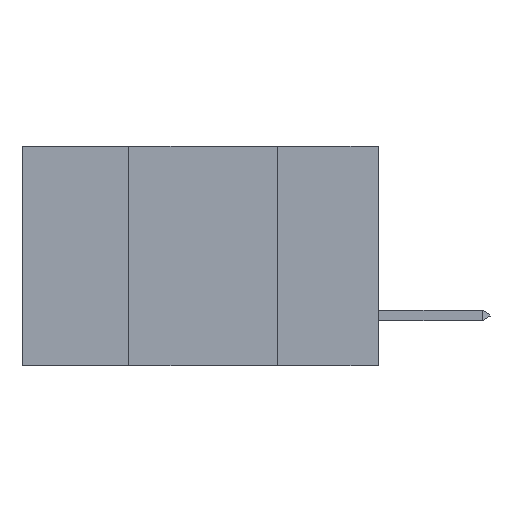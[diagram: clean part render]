
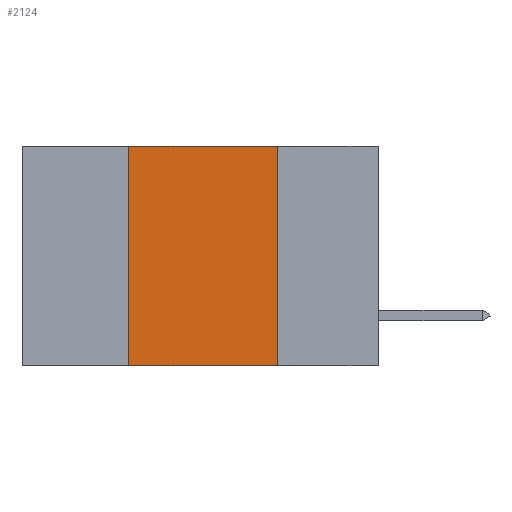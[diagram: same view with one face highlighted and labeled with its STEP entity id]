
A CAD part, left-side view. The second image highlights one B-rep face of the part: STEP entity #2124.
In plain terms, the highlighted planar face has unit normal (-1, 0, 0).
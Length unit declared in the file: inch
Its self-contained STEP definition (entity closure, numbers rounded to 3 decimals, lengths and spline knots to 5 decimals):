
#89 = ORIENTED_EDGE ( 'NONE', *, *, #5139, .F. ) ;
#172 = VERTEX_POINT ( 'NONE', #8602 ) ;
#402 = PLANE ( 'NONE',  #3498 ) ;
#580 = VECTOR ( 'NONE', #7727, 39.37008 ) ;
#938 = VECTOR ( 'NONE', #8955, 39.37008 ) ;
#2015 = EDGE_CURVE ( 'NONE', #8488, #4111, #3246, .T. ) ;
#2124 = ADVANCED_FACE ( 'NONE', ( #5912 ), #402, .F. ) ;
#2155 = CARTESIAN_POINT ( 'NONE',  ( 0., 0.17, -0.37 ) ) ;
#2163 = DIRECTION ( 'NONE',  ( 0., 0., -1. ) ) ;
#2551 = LINE ( 'NONE', #6250, #938 ) ;
#2700 = ORIENTED_EDGE ( 'NONE', *, *, #4567, .T. ) ;
#3246 = LINE ( 'NONE', #3898, #11488 ) ;
#3308 = LINE ( 'NONE', #8614, #5133 ) ;
#3342 = ORIENTED_EDGE ( 'NONE', *, *, #2015, .F. ) ;
#3453 = EDGE_LOOP ( 'NONE', ( #3342, #9810, #89, #2700 ) ) ;
#3498 = AXIS2_PLACEMENT_3D ( 'NONE', #5751, #11188, #4068 ) ;
#3898 = CARTESIAN_POINT ( 'NONE',  ( 0., 0.17, 0. ) ) ;
#4068 = DIRECTION ( 'NONE',  ( 0., 0., -1. ) ) ;
#4111 = VERTEX_POINT ( 'NONE', #2155 ) ;
#4567 = EDGE_CURVE ( 'NONE', #172, #4111, #5855, .T. ) ;
#5133 = VECTOR ( 'NONE', #8660, 39.37008 ) ;
#5139 = EDGE_CURVE ( 'NONE', #172, #8910, #3308, .T. ) ;
#5751 = CARTESIAN_POINT ( 'NONE',  ( 0., 0.6, 0. ) ) ;
#5855 = LINE ( 'NONE', #11167, #580 ) ;
#5912 = FACE_OUTER_BOUND ( 'NONE', #3453, .T. ) ;
#6250 = CARTESIAN_POINT ( 'NONE',  ( 0., 0.6, 0. ) ) ;
#6986 = EDGE_CURVE ( 'NONE', #8910, #8488, #2551, .T. ) ;
#7727 = DIRECTION ( 'NONE',  ( 0., -1., 0. ) ) ;
#8488 = VERTEX_POINT ( 'NONE', #9782 ) ;
#8602 = CARTESIAN_POINT ( 'NONE',  ( 0., 0.42, -0.37 ) ) ;
#8614 = CARTESIAN_POINT ( 'NONE',  ( 0., 0.42, 0. ) ) ;
#8660 = DIRECTION ( 'NONE',  ( 0., 0., 1. ) ) ;
#8910 = VERTEX_POINT ( 'NONE', #9761 ) ;
#8955 = DIRECTION ( 'NONE',  ( 0., -1., 0. ) ) ;
#9761 = CARTESIAN_POINT ( 'NONE',  ( 0., 0.42, 0. ) ) ;
#9782 = CARTESIAN_POINT ( 'NONE',  ( 0., 0.17, 0. ) ) ;
#9810 = ORIENTED_EDGE ( 'NONE', *, *, #6986, .F. ) ;
#11167 = CARTESIAN_POINT ( 'NONE',  ( 0., 0.6, -0.37 ) ) ;
#11188 = DIRECTION ( 'NONE',  ( 1., 0., 0. ) ) ;
#11488 = VECTOR ( 'NONE', #2163, 39.37008 ) ;
